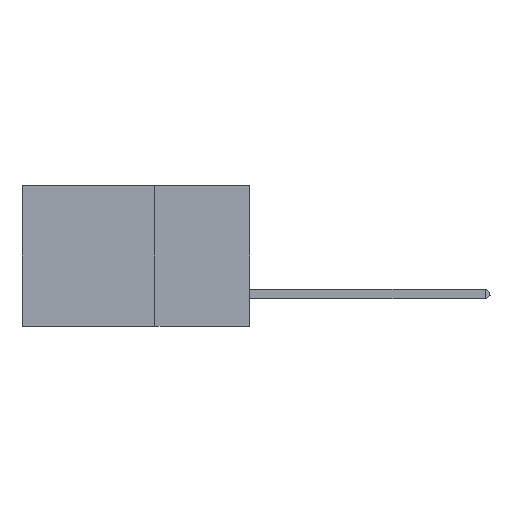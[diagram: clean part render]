
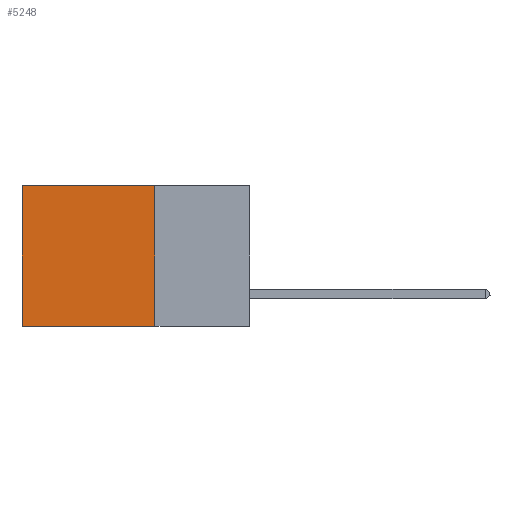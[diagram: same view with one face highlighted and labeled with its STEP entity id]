
A CAD part, left-side view. The second image highlights one B-rep face of the part: STEP entity #5248.
In plain terms, the highlighted planar face has unit normal (-1, 0, 0).
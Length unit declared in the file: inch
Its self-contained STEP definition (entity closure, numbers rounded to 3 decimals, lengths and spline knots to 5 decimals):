
#1939 = CARTESIAN_POINT ( 'NONE',  ( 0.2875, 0.25, 0. ) ) ;
#2262 = CARTESIAN_POINT ( 'NONE',  ( 0.2875, 0.25, 0. ) ) ;
#2324 = CARTESIAN_POINT ( 'NONE',  ( 0.2875, 0.6, -0.37 ) ) ;
#2738 = FACE_OUTER_BOUND ( 'NONE', #14344, .T. ) ;
#2794 = CARTESIAN_POINT ( 'NONE',  ( 0.2875, 0.25, 0. ) ) ;
#2813 = DIRECTION ( 'NONE',  ( 0., 1., 0. ) ) ;
#3104 = EDGE_CURVE ( 'NONE', #4119, #15062, #15115, .T. ) ;
#3167 = PLANE ( 'NONE',  #5457 ) ;
#3806 = DIRECTION ( 'NONE',  ( 0., 1., 0. ) ) ;
#4119 = VERTEX_POINT ( 'NONE', #10157 ) ;
#4565 = CARTESIAN_POINT ( 'NONE',  ( 0.2875, 0.25, -0.37 ) ) ;
#5248 = ADVANCED_FACE ( 'NONE', ( #2738 ), #3167, .F. ) ;
#5457 = AXIS2_PLACEMENT_3D ( 'NONE', #1939, #12772, #17343 ) ;
#5704 = VECTOR ( 'NONE', #2813, 39.37008 ) ;
#5933 = EDGE_CURVE ( 'NONE', #4119, #18084, #6343, .T. ) ;
#6343 = LINE ( 'NONE', #2262, #19811 ) ;
#6360 = ORIENTED_EDGE ( 'NONE', *, *, #13721, .T. ) ;
#7194 = VECTOR ( 'NONE', #13013, 39.37008 ) ;
#9214 = CARTESIAN_POINT ( 'NONE',  ( 0.2875, 0.25, -0.37 ) ) ;
#10157 = CARTESIAN_POINT ( 'NONE',  ( 0.2875, 0.25, 0. ) ) ;
#10198 = DIRECTION ( 'NONE',  ( 0., 0., -1. ) ) ;
#10295 = ORIENTED_EDGE ( 'NONE', *, *, #5933, .T. ) ;
#12449 = VECTOR ( 'NONE', #10198, 39.37008 ) ;
#12772 = DIRECTION ( 'NONE',  ( 1., 0., 0. ) ) ;
#13013 = DIRECTION ( 'NONE',  ( 0., 0., -1. ) ) ;
#13312 = VERTEX_POINT ( 'NONE', #2324 ) ;
#13721 = EDGE_CURVE ( 'NONE', #18084, #13312, #19165, .T. ) ;
#14344 = EDGE_LOOP ( 'NONE', ( #6360, #14450, #17660, #10295 ) ) ;
#14450 = ORIENTED_EDGE ( 'NONE', *, *, #17009, .F. ) ;
#14565 = CARTESIAN_POINT ( 'NONE',  ( 0.2875, 0.6, 0. ) ) ;
#15062 = VERTEX_POINT ( 'NONE', #9214 ) ;
#15115 = LINE ( 'NONE', #2794, #12449 ) ;
#17009 = EDGE_CURVE ( 'NONE', #15062, #13312, #17227, .T. ) ;
#17227 = LINE ( 'NONE', #4565, #5704 ) ;
#17343 = DIRECTION ( 'NONE',  ( 0., 0., -1. ) ) ;
#17660 = ORIENTED_EDGE ( 'NONE', *, *, #3104, .F. ) ;
#17661 = CARTESIAN_POINT ( 'NONE',  ( 0.2875, 0.6, 0. ) ) ;
#18084 = VERTEX_POINT ( 'NONE', #14565 ) ;
#19165 = LINE ( 'NONE', #17661, #7194 ) ;
#19811 = VECTOR ( 'NONE', #3806, 39.37008 ) ;
